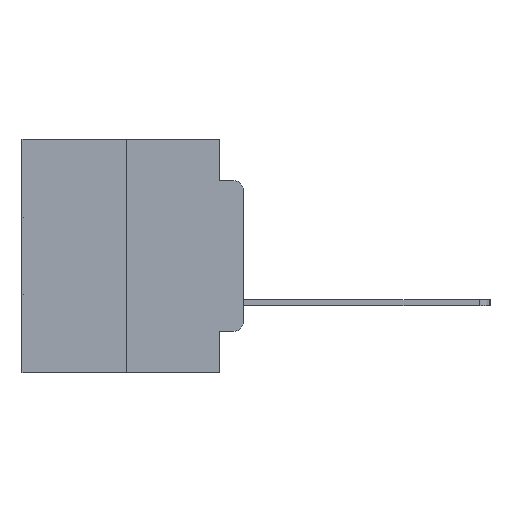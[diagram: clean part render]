
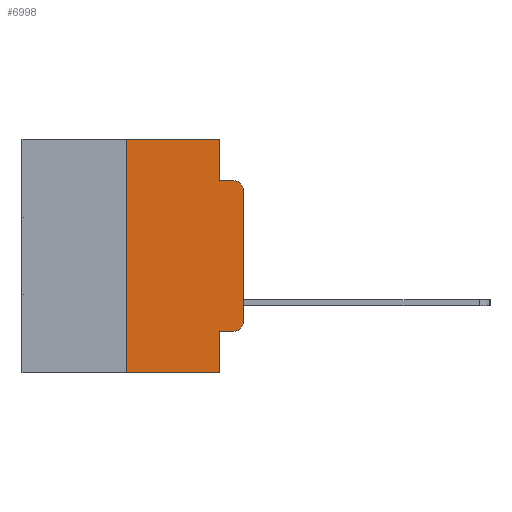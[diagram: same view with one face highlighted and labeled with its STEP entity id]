
A CAD part, left-side view. The second image highlights one B-rep face of the part: STEP entity #6998.
In plain terms, the highlighted planar face has unit normal (-1, 0, 0).
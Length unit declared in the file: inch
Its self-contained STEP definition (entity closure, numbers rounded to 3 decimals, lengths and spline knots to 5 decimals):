
#267 = CIRCLE ( 'NONE', #12470, 0.02 ) ;
#460 = DIRECTION ( 'NONE',  ( 0., 0., -1. ) ) ;
#1418 = EDGE_CURVE ( 'NONE', #8737, #14479, #11225, .T. ) ;
#1436 = CARTESIAN_POINT ( 'NONE',  ( 0., 0.25, 0. ) ) ;
#1439 = CARTESIAN_POINT ( 'NONE',  ( 0., 0.473, 0. ) ) ;
#2119 = AXIS2_PLACEMENT_3D ( 'NONE', #8373, #22189, #8474 ) ;
#2200 = CARTESIAN_POINT ( 'NONE',  ( 0., 0.02, -0.0885 ) ) ;
#2257 = CARTESIAN_POINT ( 'NONE',  ( 0., 0.051, -0.4115 ) ) ;
#3372 = VECTOR ( 'NONE', #27022, 39.37008 ) ;
#3522 = VERTEX_POINT ( 'NONE', #6799 ) ;
#3973 = DIRECTION ( 'NONE',  ( 0., -1., 0. ) ) ;
#4340 = AXIS2_PLACEMENT_3D ( 'NONE', #10695, #7171, #7141 ) ;
#4558 = EDGE_CURVE ( 'NONE', #15871, #8737, #23175, .T. ) ;
#6126 = EDGE_CURVE ( 'NONE', #15871, #19317, #27186, .T. ) ;
#6200 = PLANE ( 'NONE',  #2119 ) ;
#6600 = CARTESIAN_POINT ( 'NONE',  ( 0., 0.051, -0.0885 ) ) ;
#6799 = CARTESIAN_POINT ( 'NONE',  ( 0., 0., -0.1085 ) ) ;
#6998 = ADVANCED_FACE ( 'NONE', ( #15915 ), #6200, .F. ) ;
#7141 = DIRECTION ( 'NONE',  ( 0., 0., -1. ) ) ;
#7171 = DIRECTION ( 'NONE',  ( -1., 0., 0. ) ) ;
#7634 = EDGE_CURVE ( 'NONE', #7734, #21267, #23679, .T. ) ;
#7734 = VERTEX_POINT ( 'NONE', #16097 ) ;
#7969 = DIRECTION ( 'NONE',  ( 0., 0., 1. ) ) ;
#8030 = LINE ( 'NONE', #1439, #26181 ) ;
#8366 = CARTESIAN_POINT ( 'NONE',  ( 0., 0.051, -0.5 ) ) ;
#8373 = CARTESIAN_POINT ( 'NONE',  ( 0., 0.473, 0. ) ) ;
#8474 = DIRECTION ( 'NONE',  ( 0., 0., -1. ) ) ;
#8737 = VERTEX_POINT ( 'NONE', #15380 ) ;
#9044 = ORIENTED_EDGE ( 'NONE', *, *, #13860, .T. ) ;
#9065 = DIRECTION ( 'NONE',  ( 0., -1., 0. ) ) ;
#9188 = EDGE_CURVE ( 'NONE', #13186, #11174, #15039, .T. ) ;
#9409 = ORIENTED_EDGE ( 'NONE', *, *, #12299, .T. ) ;
#10385 = ORIENTED_EDGE ( 'NONE', *, *, #10748, .F. ) ;
#10598 = ORIENTED_EDGE ( 'NONE', *, *, #9188, .F. ) ;
#10695 = CARTESIAN_POINT ( 'NONE',  ( 0., 0.02, -0.3915 ) ) ;
#10748 = EDGE_CURVE ( 'NONE', #11174, #22742, #28201, .T. ) ;
#10928 = ORIENTED_EDGE ( 'NONE', *, *, #25785, .F. ) ;
#11174 = VERTEX_POINT ( 'NONE', #15448 ) ;
#11225 = CIRCLE ( 'NONE', #4340, 0.02 ) ;
#11441 = ORIENTED_EDGE ( 'NONE', *, *, #7634, .F. ) ;
#11899 = LINE ( 'NONE', #23869, #23302 ) ;
#12299 = EDGE_CURVE ( 'NONE', #3522, #22742, #267, .T. ) ;
#12470 = AXIS2_PLACEMENT_3D ( 'NONE', #26729, #13241, #28898 ) ;
#13186 = VERTEX_POINT ( 'NONE', #14590 ) ;
#13241 = DIRECTION ( 'NONE',  ( -1., 0., 0. ) ) ;
#13860 = EDGE_CURVE ( 'NONE', #14479, #3522, #11899, .T. ) ;
#14347 = VECTOR ( 'NONE', #16942, 39.37008 ) ;
#14479 = VERTEX_POINT ( 'NONE', #20077 ) ;
#14590 = CARTESIAN_POINT ( 'NONE',  ( 0., 0.051, 0. ) ) ;
#15039 = LINE ( 'NONE', #23685, #14347 ) ;
#15380 = CARTESIAN_POINT ( 'NONE',  ( 0., 0.02, -0.4115 ) ) ;
#15448 = CARTESIAN_POINT ( 'NONE',  ( 0., 0.051, -0.0885 ) ) ;
#15707 = CARTESIAN_POINT ( 'NONE',  ( 0., 0.25, 0. ) ) ;
#15871 = VERTEX_POINT ( 'NONE', #2257 ) ;
#15915 = FACE_OUTER_BOUND ( 'NONE', #21461, .T. ) ;
#16097 = CARTESIAN_POINT ( 'NONE',  ( 0., 0.25, -0.5 ) ) ;
#16243 = ORIENTED_EDGE ( 'NONE', *, *, #25420, .T. ) ;
#16942 = DIRECTION ( 'NONE',  ( 0., 0., -1. ) ) ;
#17130 = VECTOR ( 'NONE', #9065, 39.37008 ) ;
#17751 = CARTESIAN_POINT ( 'NONE',  ( 0., 0.473, -0.5 ) ) ;
#18830 = VECTOR ( 'NONE', #3973, 39.37008 ) ;
#18949 = CARTESIAN_POINT ( 'NONE',  ( 0., 0.051, 0. ) ) ;
#19317 = VERTEX_POINT ( 'NONE', #8366 ) ;
#19777 = ORIENTED_EDGE ( 'NONE', *, *, #6126, .F. ) ;
#20077 = CARTESIAN_POINT ( 'NONE',  ( 0., 0., -0.3915 ) ) ;
#21009 = ORIENTED_EDGE ( 'NONE', *, *, #4558, .T. ) ;
#21267 = VERTEX_POINT ( 'NONE', #1436 ) ;
#21278 = VECTOR ( 'NONE', #460, 39.37008 ) ;
#21324 = ORIENTED_EDGE ( 'NONE', *, *, #1418, .T. ) ;
#21461 = EDGE_LOOP ( 'NONE', ( #9044, #9409, #10385, #10598, #10928, #11441, #16243, #19777, #21009, #21324 ) ) ;
#22189 = DIRECTION ( 'NONE',  ( 1., 0., 0. ) ) ;
#22742 = VERTEX_POINT ( 'NONE', #2200 ) ;
#23175 = LINE ( 'NONE', #25210, #17130 ) ;
#23302 = VECTOR ( 'NONE', #7969, 39.37008 ) ;
#23679 = LINE ( 'NONE', #15707, #27431 ) ;
#23685 = CARTESIAN_POINT ( 'NONE',  ( 0., 0.051, 0. ) ) ;
#23869 = CARTESIAN_POINT ( 'NONE',  ( 0., 0., 0. ) ) ;
#24150 = LINE ( 'NONE', #17751, #18830 ) ;
#25210 = CARTESIAN_POINT ( 'NONE',  ( 0., 0.051, -0.4115 ) ) ;
#25420 = EDGE_CURVE ( 'NONE', #7734, #19317, #24150, .T. ) ;
#25785 = EDGE_CURVE ( 'NONE', #21267, #13186, #8030, .T. ) ;
#26181 = VECTOR ( 'NONE', #28765, 39.37008 ) ;
#26729 = CARTESIAN_POINT ( 'NONE',  ( 0., 0.02, -0.1085 ) ) ;
#26893 = DIRECTION ( 'NONE',  ( 0., 0., 1. ) ) ;
#27022 = DIRECTION ( 'NONE',  ( 0., -1., 0. ) ) ;
#27186 = LINE ( 'NONE', #18949, #21278 ) ;
#27431 = VECTOR ( 'NONE', #26893, 39.37008 ) ;
#28201 = LINE ( 'NONE', #6600, #3372 ) ;
#28765 = DIRECTION ( 'NONE',  ( 0., -1., 0. ) ) ;
#28898 = DIRECTION ( 'NONE',  ( 0., 0., -1. ) ) ;
